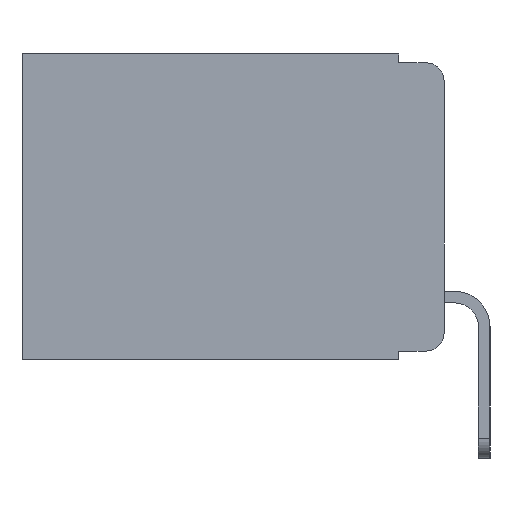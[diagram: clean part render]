
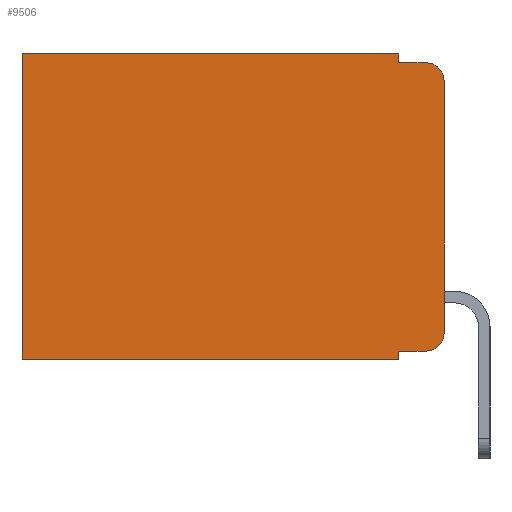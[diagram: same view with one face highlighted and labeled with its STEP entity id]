
A CAD part, left-side view. The second image highlights one B-rep face of the part: STEP entity #9506.
In plain terms, the highlighted planar face has unit normal (-1, 0, 0).
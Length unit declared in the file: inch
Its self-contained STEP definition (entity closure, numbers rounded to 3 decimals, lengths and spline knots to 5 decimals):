
#459 = CARTESIAN_POINT ( 'NONE',  ( 0.298, 0.02, -0.03 ) ) ;
#620 = CARTESIAN_POINT ( 'NONE',  ( 0.298, 0.051, -0.333 ) ) ;
#704 = DIRECTION ( 'NONE',  ( -1., 0., 0. ) ) ;
#1158 = VECTOR ( 'NONE', #14164, 39.37008 ) ;
#1216 = CARTESIAN_POINT ( 'NONE',  ( 0.298, 0.051, 0. ) ) ;
#1871 = ORIENTED_EDGE ( 'NONE', *, *, #8665, .F. ) ;
#1946 = VERTEX_POINT ( 'NONE', #9679 ) ;
#2236 = LINE ( 'NONE', #17974, #13783 ) ;
#2247 = DIRECTION ( 'NONE',  ( 0., 0., -1. ) ) ;
#2307 = CARTESIAN_POINT ( 'NONE',  ( 0.298, 0.473, 0. ) ) ;
#2866 = LINE ( 'NONE', #17249, #6539 ) ;
#3169 = CARTESIAN_POINT ( 'NONE',  ( 0.298, 0., -0.03 ) ) ;
#3482 = EDGE_CURVE ( 'NONE', #7283, #1946, #2866, .T. ) ;
#3539 = PLANE ( 'NONE',  #14866 ) ;
#3888 = DIRECTION ( 'NONE',  ( 0., 0., -1. ) ) ;
#3947 = VECTOR ( 'NONE', #13039, 39.37008 ) ;
#4428 = CIRCLE ( 'NONE', #12318, 0.02 ) ;
#4920 = VECTOR ( 'NONE', #3888, 39.37008 ) ;
#4996 = VERTEX_POINT ( 'NONE', #4997 ) ;
#4997 = CARTESIAN_POINT ( 'NONE',  ( 0.298, 0.02, -0.01 ) ) ;
#5124 = DIRECTION ( 'NONE',  ( 0., 0., -1. ) ) ;
#6539 = VECTOR ( 'NONE', #17878, 39.37008 ) ;
#6585 = ORIENTED_EDGE ( 'NONE', *, *, #8640, .T. ) ;
#7283 = VERTEX_POINT ( 'NONE', #1216 ) ;
#7673 = CARTESIAN_POINT ( 'NONE',  ( 0.298, 0.051, -0.333 ) ) ;
#8104 = LINE ( 'NONE', #620, #3947 ) ;
#8260 = ORIENTED_EDGE ( 'NONE', *, *, #8667, .T. ) ;
#8327 = AXIS2_PLACEMENT_3D ( 'NONE', #459, #11489, #2247 ) ;
#8339 = EDGE_CURVE ( 'NONE', #12806, #14321, #14001, .T. ) ;
#8633 = EDGE_CURVE ( 'NONE', #15429, #15476, #2236, .T. ) ;
#8640 = EDGE_CURVE ( 'NONE', #15429, #4996, #10021, .T. ) ;
#8661 = EDGE_CURVE ( 'NONE', #10055, #4996, #9556, .T. ) ;
#8665 = EDGE_CURVE ( 'NONE', #7283, #10055, #13373, .T. ) ;
#8667 = EDGE_CURVE ( 'NONE', #1946, #14321, #16385, .T. ) ;
#8668 = EDGE_CURVE ( 'NONE', #18500, #12806, #9084, .T. ) ;
#8692 = EDGE_CURVE ( 'NONE', #18500, #10750, #8104, .T. ) ;
#8694 = EDGE_CURVE ( 'NONE', #10750, #15476, #4428, .T. ) ;
#9084 = LINE ( 'NONE', #14278, #15991 ) ;
#9435 = CARTESIAN_POINT ( 'NONE',  ( 0.298, 0., -0.313 ) ) ;
#9506 = ADVANCED_FACE ( 'NONE', ( #14143 ), #3539, .F. ) ;
#9556 = LINE ( 'NONE', #15507, #1158 ) ;
#9679 = CARTESIAN_POINT ( 'NONE',  ( 0.298, 0.473, 0. ) ) ;
#10021 = CIRCLE ( 'NONE', #8327, 0.02 ) ;
#10055 = VERTEX_POINT ( 'NONE', #16608 ) ;
#10059 = CARTESIAN_POINT ( 'NONE',  ( 0.298, 0.051, 0. ) ) ;
#10184 = CARTESIAN_POINT ( 'NONE',  ( 0.298, 0.02, -0.313 ) ) ;
#10750 = VERTEX_POINT ( 'NONE', #13591 ) ;
#11489 = DIRECTION ( 'NONE',  ( -1., 0., 0. ) ) ;
#11545 = DIRECTION ( 'NONE',  ( 0., 0., -1. ) ) ;
#11679 = DIRECTION ( 'NONE',  ( 0., 0., -1. ) ) ;
#12318 = AXIS2_PLACEMENT_3D ( 'NONE', #10184, #704, #11679 ) ;
#12473 = CARTESIAN_POINT ( 'NONE',  ( 0.298, 0.473, -0.343 ) ) ;
#12660 = ORIENTED_EDGE ( 'NONE', *, *, #8694, .T. ) ;
#12680 = ORIENTED_EDGE ( 'NONE', *, *, #3482, .T. ) ;
#12806 = VERTEX_POINT ( 'NONE', #17307 ) ;
#12818 = EDGE_LOOP ( 'NONE', ( #13481, #6585, #16329, #1871, #12680, #8260, #17900, #13695, #13283, #12660 ) ) ;
#12877 = DIRECTION ( 'NONE',  ( 0., 0., -1. ) ) ;
#12976 = VECTOR ( 'NONE', #11545, 39.37008 ) ;
#13039 = DIRECTION ( 'NONE',  ( 0., -1., 0. ) ) ;
#13283 = ORIENTED_EDGE ( 'NONE', *, *, #8692, .T. ) ;
#13373 = LINE ( 'NONE', #10059, #12976 ) ;
#13481 = ORIENTED_EDGE ( 'NONE', *, *, #8633, .F. ) ;
#13558 = CARTESIAN_POINT ( 'NONE',  ( 0.298, 0., -0.343 ) ) ;
#13591 = CARTESIAN_POINT ( 'NONE',  ( 0.298, 0.02, -0.333 ) ) ;
#13695 = ORIENTED_EDGE ( 'NONE', *, *, #8668, .F. ) ;
#13783 = VECTOR ( 'NONE', #12877, 39.37008 ) ;
#14001 = LINE ( 'NONE', #13558, #16994 ) ;
#14002 = DIRECTION ( 'NONE',  ( 1., 0., 0. ) ) ;
#14143 = FACE_OUTER_BOUND ( 'NONE', #12818, .T. ) ;
#14164 = DIRECTION ( 'NONE',  ( 0., -1., 0. ) ) ;
#14278 = CARTESIAN_POINT ( 'NONE',  ( 0.298, 0.051, 0. ) ) ;
#14321 = VERTEX_POINT ( 'NONE', #12473 ) ;
#14856 = DIRECTION ( 'NONE',  ( 0., 1., 0. ) ) ;
#14866 = AXIS2_PLACEMENT_3D ( 'NONE', #17806, #14002, #5124 ) ;
#15429 = VERTEX_POINT ( 'NONE', #3169 ) ;
#15476 = VERTEX_POINT ( 'NONE', #9435 ) ;
#15507 = CARTESIAN_POINT ( 'NONE',  ( 0.298, 0.051, -0.01 ) ) ;
#15563 = DIRECTION ( 'NONE',  ( 0., 0., -1. ) ) ;
#15991 = VECTOR ( 'NONE', #15563, 39.37008 ) ;
#16329 = ORIENTED_EDGE ( 'NONE', *, *, #8661, .F. ) ;
#16385 = LINE ( 'NONE', #2307, #4920 ) ;
#16608 = CARTESIAN_POINT ( 'NONE',  ( 0.298, 0.051, -0.01 ) ) ;
#16994 = VECTOR ( 'NONE', #14856, 39.37008 ) ;
#17249 = CARTESIAN_POINT ( 'NONE',  ( 0.298, 0., 0. ) ) ;
#17307 = CARTESIAN_POINT ( 'NONE',  ( 0.298, 0.051, -0.343 ) ) ;
#17806 = CARTESIAN_POINT ( 'NONE',  ( 0.298, 0., 0. ) ) ;
#17878 = DIRECTION ( 'NONE',  ( 0., 1., 0. ) ) ;
#17900 = ORIENTED_EDGE ( 'NONE', *, *, #8339, .F. ) ;
#17974 = CARTESIAN_POINT ( 'NONE',  ( 0.298, 0., 0. ) ) ;
#18500 = VERTEX_POINT ( 'NONE', #7673 ) ;
